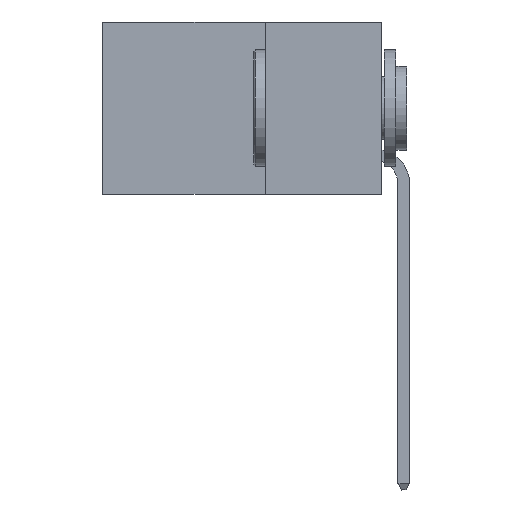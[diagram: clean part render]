
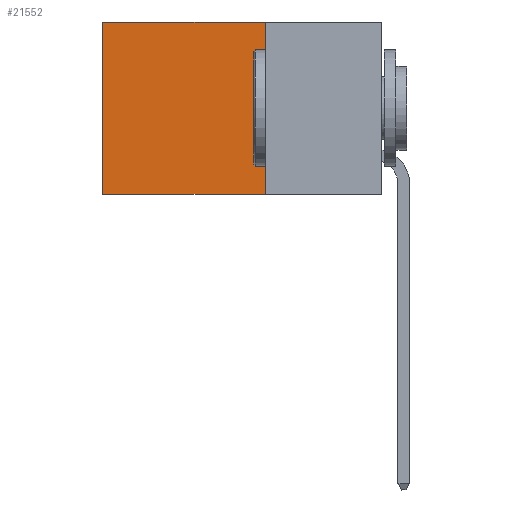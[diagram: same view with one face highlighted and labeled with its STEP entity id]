
A CAD part, left-side view. The second image highlights one B-rep face of the part: STEP entity #21552.
In plain terms, the highlighted planar face has unit normal (-1, 0, 0).
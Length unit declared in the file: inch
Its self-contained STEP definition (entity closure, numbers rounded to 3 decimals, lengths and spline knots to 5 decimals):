
#1515 = CARTESIAN_POINT ( 'NONE',  ( 0.2875, 0.25, -0.37 ) ) ;
#3242 = CARTESIAN_POINT ( 'NONE',  ( 0.2875, 0.25, 0. ) ) ;
#4252 = CARTESIAN_POINT ( 'NONE',  ( 0.2875, 0.25, 0. ) ) ;
#5297 = CARTESIAN_POINT ( 'NONE',  ( 0.2875, 0.25, -0.37 ) ) ;
#6009 = CARTESIAN_POINT ( 'NONE',  ( 0.2875, 0.6, -0.37 ) ) ;
#6814 = DIRECTION ( 'NONE',  ( 1., 0., 0. ) ) ;
#6855 = AXIS2_PLACEMENT_3D ( 'NONE', #18639, #6814, #13892 ) ;
#7092 = VECTOR ( 'NONE', #28516, 39.37008 ) ;
#7305 = VERTEX_POINT ( 'NONE', #28504 ) ;
#7394 = VERTEX_POINT ( 'NONE', #1515 ) ;
#8958 = ORIENTED_EDGE ( 'NONE', *, *, #22745, .T. ) ;
#9513 = VECTOR ( 'NONE', #29650, 39.37008 ) ;
#11412 = EDGE_CURVE ( 'NONE', #28839, #7394, #22336, .T. ) ;
#13279 = LINE ( 'NONE', #5297, #7092 ) ;
#13892 = DIRECTION ( 'NONE',  ( 0., 0., -1. ) ) ;
#13978 = PLANE ( 'NONE',  #6855 ) ;
#15109 = EDGE_CURVE ( 'NONE', #7394, #26737, #13279, .T. ) ;
#15541 = ORIENTED_EDGE ( 'NONE', *, *, #15109, .F. ) ;
#17881 = FACE_OUTER_BOUND ( 'NONE', #25207, .T. ) ;
#18639 = CARTESIAN_POINT ( 'NONE',  ( 0.2875, 0.25, 0. ) ) ;
#21552 = ADVANCED_FACE ( 'NONE', ( #17881 ), #13978, .F. ) ;
#21961 = VECTOR ( 'NONE', #23871, 39.37008 ) ;
#22336 = LINE ( 'NONE', #3242, #21961 ) ;
#22745 = EDGE_CURVE ( 'NONE', #7305, #26737, #27573, .T. ) ;
#22940 = CARTESIAN_POINT ( 'NONE',  ( 0.2875, 0.6, 0. ) ) ;
#23019 = DIRECTION ( 'NONE',  ( 0., 0., -1. ) ) ;
#23172 = EDGE_CURVE ( 'NONE', #28839, #7305, #25760, .T. ) ;
#23871 = DIRECTION ( 'NONE',  ( 0., 0., -1. ) ) ;
#24990 = ORIENTED_EDGE ( 'NONE', *, *, #11412, .F. ) ;
#25207 = EDGE_LOOP ( 'NONE', ( #8958, #15541, #24990, #28024 ) ) ;
#25760 = LINE ( 'NONE', #26530, #9513 ) ;
#26530 = CARTESIAN_POINT ( 'NONE',  ( 0.2875, 0.25, 0. ) ) ;
#26737 = VERTEX_POINT ( 'NONE', #6009 ) ;
#27573 = LINE ( 'NONE', #22940, #28318 ) ;
#28024 = ORIENTED_EDGE ( 'NONE', *, *, #23172, .T. ) ;
#28318 = VECTOR ( 'NONE', #23019, 39.37008 ) ;
#28504 = CARTESIAN_POINT ( 'NONE',  ( 0.2875, 0.6, 0. ) ) ;
#28516 = DIRECTION ( 'NONE',  ( 0., 1., 0. ) ) ;
#28839 = VERTEX_POINT ( 'NONE', #4252 ) ;
#29650 = DIRECTION ( 'NONE',  ( 0., 1., 0. ) ) ;
